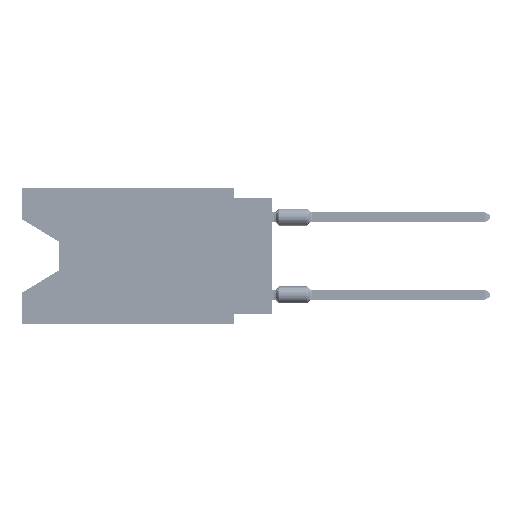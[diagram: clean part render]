
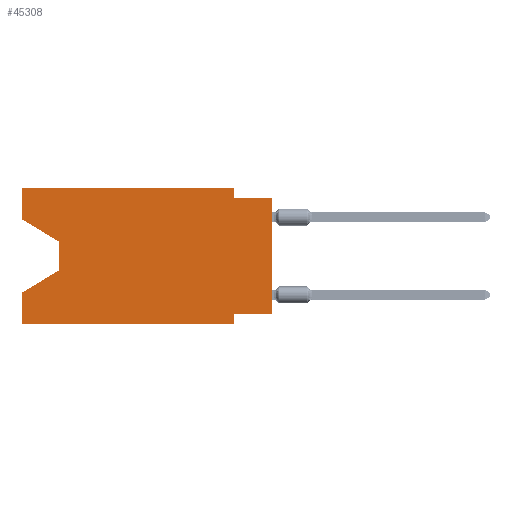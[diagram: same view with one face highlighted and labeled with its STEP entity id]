
A CAD part, left-side view. The second image highlights one B-rep face of the part: STEP entity #45308.
In plain terms, the highlighted planar face has unit normal (-1, 0, 0).
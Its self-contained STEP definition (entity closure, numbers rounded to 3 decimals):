
#61 = AXIS2_PLACEMENT_3D ( 'NONE', #74062, #9258, #66242 ) ;
#891 = VECTOR ( 'NONE', #23130, 1000. ) ;
#1392 = CARTESIAN_POINT ( 'NONE',  ( 0., 16.383, 0. ) ) ;
#1675 = VERTEX_POINT ( 'NONE', #61114 ) ;
#2330 = VERTEX_POINT ( 'NONE', #74739 ) ;
#3232 = LINE ( 'NONE', #38683, #107581 ) ;
#4699 = EDGE_CURVE ( 'NONE', #33869, #107883, #62100, .T. ) ;
#9258 = DIRECTION ( 'NONE',  ( 1., 0., 0. ) ) ;
#12304 = CARTESIAN_POINT ( 'NONE',  ( 0., 16.383, 0. ) ) ;
#14327 = DIRECTION ( 'NONE',  ( 0., -1., 0. ) ) ;
#16508 = DIRECTION ( 'NONE',  ( 0., 0., -1. ) ) ;
#18416 = EDGE_CURVE ( 'NONE', #91600, #54830, #46596, .T. ) ;
#19164 = CARTESIAN_POINT ( 'NONE',  ( 0., 13.97, -5.385 ) ) ;
#19167 = VECTOR ( 'NONE', #82042, 1000. ) ;
#19844 = VECTOR ( 'NONE', #65118, 1000. ) ;
#20056 = LINE ( 'NONE', #1392, #90355 ) ;
#21068 = VERTEX_POINT ( 'NONE', #64362 ) ;
#23130 = DIRECTION ( 'NONE',  ( 0., -1., 0. ) ) ;
#28511 = DIRECTION ( 'NONE',  ( 0., -0.855, -0.519 ) ) ;
#29481 = DIRECTION ( 'NONE',  ( 0., -1., 0. ) ) ;
#32111 = LINE ( 'NONE', #105322, #891 ) ;
#33869 = VERTEX_POINT ( 'NONE', #38617 ) ;
#34274 = ORIENTED_EDGE ( 'NONE', *, *, #4699, .T. ) ;
#34810 = CARTESIAN_POINT ( 'NONE',  ( 0., 0., -8.255 ) ) ;
#35486 = ORIENTED_EDGE ( 'NONE', *, *, #51824, .F. ) ;
#36762 = CARTESIAN_POINT ( 'NONE',  ( 0., 2.54, 0. ) ) ;
#38617 = CARTESIAN_POINT ( 'NONE',  ( 0., 13.97, -3.505 ) ) ;
#38683 = CARTESIAN_POINT ( 'NONE',  ( 0., 16.383, -2.038 ) ) ;
#39469 = ORIENTED_EDGE ( 'NONE', *, *, #80221, .T. ) ;
#42150 = ORIENTED_EDGE ( 'NONE', *, *, #51282, .T. ) ;
#42247 = EDGE_CURVE ( 'NONE', #21068, #112911, #45747, .T. ) ;
#42516 = LINE ( 'NONE', #69541, #59766 ) ;
#43757 = ORIENTED_EDGE ( 'NONE', *, *, #114766, .F. ) ;
#44064 = VERTEX_POINT ( 'NONE', #34810 ) ;
#45308 = ADVANCED_FACE ( 'NONE', ( #46448 ), #102273, .F. ) ;
#45747 = LINE ( 'NONE', #83544, #105030 ) ;
#46448 = FACE_OUTER_BOUND ( 'NONE', #65514, .T. ) ;
#46596 = LINE ( 'NONE', #83214, #19167 ) ;
#47098 = VECTOR ( 'NONE', #109795, 1000. ) ;
#49735 = ORIENTED_EDGE ( 'NONE', *, *, #57780, .T. ) ;
#51282 = EDGE_CURVE ( 'NONE', #1675, #112911, #32111, .T. ) ;
#51488 = CARTESIAN_POINT ( 'NONE',  ( 0., 0., 0. ) ) ;
#51824 = EDGE_CURVE ( 'NONE', #54830, #95469, #111692, .T. ) ;
#51991 = CARTESIAN_POINT ( 'NONE',  ( 0., 13.97, -5.385 ) ) ;
#54830 = VERTEX_POINT ( 'NONE', #90852 ) ;
#55447 = ORIENTED_EDGE ( 'NONE', *, *, #75447, .T. ) ;
#56476 = CARTESIAN_POINT ( 'NONE',  ( 0., 16.383, 0. ) ) ;
#57780 = EDGE_CURVE ( 'NONE', #44064, #95469, #106727, .T. ) ;
#59766 = VECTOR ( 'NONE', #14327, 1000. ) ;
#61114 = CARTESIAN_POINT ( 'NONE',  ( 0., 16.383, -8.89 ) ) ;
#62100 = LINE ( 'NONE', #98737, #100998 ) ;
#63939 = CARTESIAN_POINT ( 'NONE',  ( 0., 0., -0.635 ) ) ;
#64362 = CARTESIAN_POINT ( 'NONE',  ( 0., 2.54, -8.255 ) ) ;
#65118 = DIRECTION ( 'NONE',  ( 0., 1., 0. ) ) ;
#65452 = CARTESIAN_POINT ( 'NONE',  ( 0., 16.383, -2.038 ) ) ;
#65514 = EDGE_LOOP ( 'NONE', ( #55447, #34274, #39469, #43757, #42150, #115462, #113165, #49735, #35486, #78713, #78732, #84128 ) ) ;
#66242 = DIRECTION ( 'NONE',  ( 0., 0., -1. ) ) ;
#69169 = EDGE_CURVE ( 'NONE', #86806, #117892, #102128, .T. ) ;
#69541 = CARTESIAN_POINT ( 'NONE',  ( 0., 16.383, 0. ) ) ;
#74062 = CARTESIAN_POINT ( 'NONE',  ( 0., 16.383, 0. ) ) ;
#74739 = CARTESIAN_POINT ( 'NONE',  ( 0., 16.383, -6.852 ) ) ;
#75447 = EDGE_CURVE ( 'NONE', #86806, #33869, #3232, .T. ) ;
#78713 = ORIENTED_EDGE ( 'NONE', *, *, #18416, .F. ) ;
#78732 = ORIENTED_EDGE ( 'NONE', *, *, #94713, .F. ) ;
#80221 = EDGE_CURVE ( 'NONE', #107883, #2330, #118185, .T. ) ;
#82042 = DIRECTION ( 'NONE',  ( 0., 0., -1. ) ) ;
#82322 = CARTESIAN_POINT ( 'NONE',  ( 0., 0., -0.635 ) ) ;
#82383 = DIRECTION ( 'NONE',  ( 0., 0., -1. ) ) ;
#83124 = LINE ( 'NONE', #109560, #19844 ) ;
#83214 = CARTESIAN_POINT ( 'NONE',  ( 0., 2.54, 0. ) ) ;
#83544 = CARTESIAN_POINT ( 'NONE',  ( 0., 2.54, -8.89 ) ) ;
#84128 = ORIENTED_EDGE ( 'NONE', *, *, #69169, .F. ) ;
#86806 = VERTEX_POINT ( 'NONE', #65452 ) ;
#88138 = DIRECTION ( 'NONE',  ( 0., 0., 1. ) ) ;
#90355 = VECTOR ( 'NONE', #113035, 1000. ) ;
#90852 = CARTESIAN_POINT ( 'NONE',  ( 0., 2.54, -0.635 ) ) ;
#91600 = VERTEX_POINT ( 'NONE', #36762 ) ;
#93116 = DIRECTION ( 'NONE',  ( 0., 0., 1. ) ) ;
#94713 = EDGE_CURVE ( 'NONE', #117892, #91600, #42516, .T. ) ;
#95469 = VERTEX_POINT ( 'NONE', #63939 ) ;
#98737 = CARTESIAN_POINT ( 'NONE',  ( 0., 13.97, -3.505 ) ) ;
#100998 = VECTOR ( 'NONE', #16508, 1000. ) ;
#101896 = VECTOR ( 'NONE', #88138, 1000. ) ;
#102128 = LINE ( 'NONE', #56476, #106639 ) ;
#102273 = PLANE ( 'NONE',  #61 ) ;
#104881 = EDGE_CURVE ( 'NONE', #44064, #21068, #83124, .T. ) ;
#105030 = VECTOR ( 'NONE', #82383, 1000. ) ;
#105322 = CARTESIAN_POINT ( 'NONE',  ( 0., 16.383, -8.89 ) ) ;
#106639 = VECTOR ( 'NONE', #93116, 1000. ) ;
#106727 = LINE ( 'NONE', #51488, #101896 ) ;
#107581 = VECTOR ( 'NONE', #28511, 1000. ) ;
#107883 = VERTEX_POINT ( 'NONE', #51991 ) ;
#109560 = CARTESIAN_POINT ( 'NONE',  ( 0., 0., -8.255 ) ) ;
#109795 = DIRECTION ( 'NONE',  ( 0., 0.855, -0.519 ) ) ;
#110631 = CARTESIAN_POINT ( 'NONE',  ( 0., 2.54, -8.89 ) ) ;
#111692 = LINE ( 'NONE', #82322, #116002 ) ;
#112911 = VERTEX_POINT ( 'NONE', #110631 ) ;
#113035 = DIRECTION ( 'NONE',  ( 0., 0., 1. ) ) ;
#113165 = ORIENTED_EDGE ( 'NONE', *, *, #104881, .F. ) ;
#114766 = EDGE_CURVE ( 'NONE', #1675, #2330, #20056, .T. ) ;
#115462 = ORIENTED_EDGE ( 'NONE', *, *, #42247, .F. ) ;
#116002 = VECTOR ( 'NONE', #29481, 1000. ) ;
#117892 = VERTEX_POINT ( 'NONE', #12304 ) ;
#118185 = LINE ( 'NONE', #19164, #47098 ) ;
